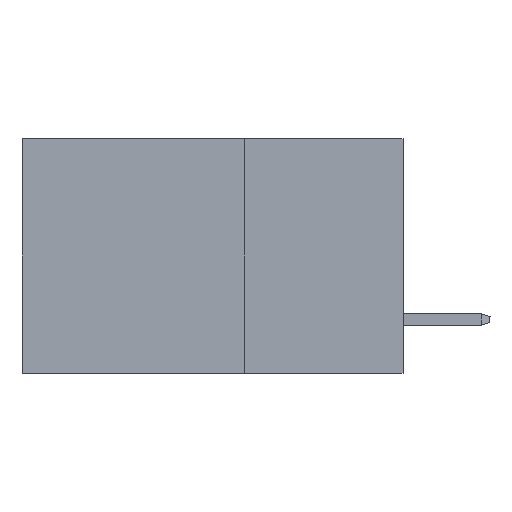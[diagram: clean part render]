
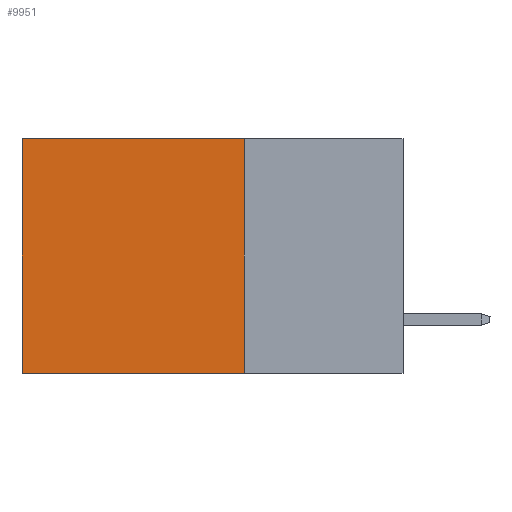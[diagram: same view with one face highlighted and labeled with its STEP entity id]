
A CAD part, left-side view. The second image highlights one B-rep face of the part: STEP entity #9951.
In plain terms, the highlighted planar face has unit normal (-1, 0, 0).
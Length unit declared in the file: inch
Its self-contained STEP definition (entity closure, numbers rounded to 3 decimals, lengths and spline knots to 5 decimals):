
#18 = VECTOR ( 'NONE', #11637, 39.37008 ) ;
#105 = EDGE_CURVE ( 'NONE', #10792, #10746, #5968, .T. ) ;
#1041 = VECTOR ( 'NONE', #1231, 39.37008 ) ;
#1231 = DIRECTION ( 'NONE',  ( 0., 0., -1. ) ) ;
#1874 = DIRECTION ( 'NONE',  ( 0., 0., -1. ) ) ;
#1979 = ORIENTED_EDGE ( 'NONE', *, *, #105, .T. ) ;
#2000 = CARTESIAN_POINT ( 'NONE',  ( 0.2875, 0.6, -0.37 ) ) ;
#2074 = LINE ( 'NONE', #12516, #18 ) ;
#2084 = CARTESIAN_POINT ( 'NONE',  ( 0.2875, 0.25, 0. ) ) ;
#2172 = ORIENTED_EDGE ( 'NONE', *, *, #10280, .F. ) ;
#2584 = VECTOR ( 'NONE', #4893, 39.37008 ) ;
#2915 = FACE_OUTER_BOUND ( 'NONE', #12293, .T. ) ;
#3663 = CARTESIAN_POINT ( 'NONE',  ( 0.2875, 0.25, -0.37 ) ) ;
#3835 = VERTEX_POINT ( 'NONE', #2000 ) ;
#4032 = DIRECTION ( 'NONE',  ( 1., 0., 0. ) ) ;
#4428 = VECTOR ( 'NONE', #9889, 39.37008 ) ;
#4893 = DIRECTION ( 'NONE',  ( 0., 1., 0. ) ) ;
#5968 = LINE ( 'NONE', #8153, #2584 ) ;
#6725 = LINE ( 'NONE', #3663, #4428 ) ;
#6959 = PLANE ( 'NONE',  #11866 ) ;
#7448 = CARTESIAN_POINT ( 'NONE',  ( 0.2875, 0.25, -0.37 ) ) ;
#8153 = CARTESIAN_POINT ( 'NONE',  ( 0.2875, 0.25, 0. ) ) ;
#8982 = VERTEX_POINT ( 'NONE', #7448 ) ;
#9099 = EDGE_CURVE ( 'NONE', #8982, #3835, #6725, .T. ) ;
#9889 = DIRECTION ( 'NONE',  ( 0., 1., 0. ) ) ;
#9951 = ADVANCED_FACE ( 'NONE', ( #2915 ), #6959, .F. ) ;
#10187 = CARTESIAN_POINT ( 'NONE',  ( 0.2875, 0.6, 0. ) ) ;
#10280 = EDGE_CURVE ( 'NONE', #10792, #8982, #12572, .T. ) ;
#10746 = VERTEX_POINT ( 'NONE', #10187 ) ;
#10792 = VERTEX_POINT ( 'NONE', #2084 ) ;
#10986 = CARTESIAN_POINT ( 'NONE',  ( 0.2875, 0.25, 0. ) ) ;
#11561 = ORIENTED_EDGE ( 'NONE', *, *, #9099, .F. ) ;
#11637 = DIRECTION ( 'NONE',  ( 0., 0., -1. ) ) ;
#11838 = EDGE_CURVE ( 'NONE', #10746, #3835, #2074, .T. ) ;
#11866 = AXIS2_PLACEMENT_3D ( 'NONE', #10986, #4032, #1874 ) ;
#12293 = EDGE_LOOP ( 'NONE', ( #12811, #11561, #2172, #1979 ) ) ;
#12446 = CARTESIAN_POINT ( 'NONE',  ( 0.2875, 0.25, 0. ) ) ;
#12516 = CARTESIAN_POINT ( 'NONE',  ( 0.2875, 0.6, 0. ) ) ;
#12572 = LINE ( 'NONE', #12446, #1041 ) ;
#12811 = ORIENTED_EDGE ( 'NONE', *, *, #11838, .T. ) ;
